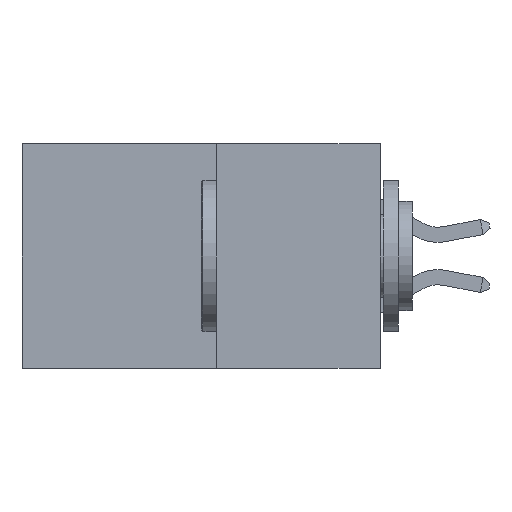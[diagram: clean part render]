
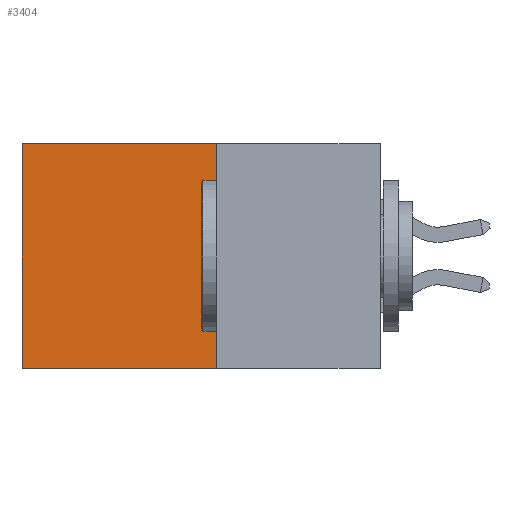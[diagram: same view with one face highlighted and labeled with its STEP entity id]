
A CAD part, left-side view. The second image highlights one B-rep face of the part: STEP entity #3404.
In plain terms, the highlighted planar face has unit normal (-1, 0, 0).
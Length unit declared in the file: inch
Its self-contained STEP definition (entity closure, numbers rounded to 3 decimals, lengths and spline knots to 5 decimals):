
#109 = CARTESIAN_POINT ( 'NONE',  ( 0.277, 0.27, 0. ) ) ;
#290 = DIRECTION ( 'NONE',  ( 0., 1., 0. ) ) ;
#427 = CARTESIAN_POINT ( 'NONE',  ( 0.277, 0.27, -0.37 ) ) ;
#1218 = CARTESIAN_POINT ( 'NONE',  ( 0.277, 0.59, -0.37 ) ) ;
#1622 = CARTESIAN_POINT ( 'NONE',  ( 0.277, 0.59, -0.37 ) ) ;
#3404 = ADVANCED_FACE ( 'NONE', ( #16937 ), #18128, .F. ) ;
#3435 = DIRECTION ( 'NONE',  ( 0., 0., -1. ) ) ;
#5692 = ORIENTED_EDGE ( 'NONE', *, *, #20741, .T. ) ;
#5983 = LINE ( 'NONE', #10711, #20294 ) ;
#6205 = LINE ( 'NONE', #1622, #21079 ) ;
#8335 = ORIENTED_EDGE ( 'NONE', *, *, #9050, .F. ) ;
#8453 = VECTOR ( 'NONE', #15107, 39.37008 ) ;
#9037 = LINE ( 'NONE', #109, #8453 ) ;
#9050 = EDGE_CURVE ( 'NONE', #17726, #15517, #5983, .T. ) ;
#9116 = DIRECTION ( 'NONE',  ( 0., 0., -1. ) ) ;
#9784 = VERTEX_POINT ( 'NONE', #23507 ) ;
#9999 = LINE ( 'NONE', #427, #14352 ) ;
#10662 = EDGE_CURVE ( 'NONE', #15517, #20587, #9999, .T. ) ;
#10711 = CARTESIAN_POINT ( 'NONE',  ( 0.277, 0.27, -0.37 ) ) ;
#13390 = EDGE_CURVE ( 'NONE', #17726, #9784, #9037, .T. ) ;
#13957 = ORIENTED_EDGE ( 'NONE', *, *, #10662, .F. ) ;
#14024 = ORIENTED_EDGE ( 'NONE', *, *, #13390, .T. ) ;
#14352 = VECTOR ( 'NONE', #290, 39.37008 ) ;
#15107 = DIRECTION ( 'NONE',  ( 0., 1., 0. ) ) ;
#15517 = VERTEX_POINT ( 'NONE', #19638 ) ;
#16448 = CARTESIAN_POINT ( 'NONE',  ( 0.277, 0.27, -0.37 ) ) ;
#16605 = DIRECTION ( 'NONE',  ( 0., 0., -1. ) ) ;
#16923 = DIRECTION ( 'NONE',  ( 1., 0., 0. ) ) ;
#16937 = FACE_OUTER_BOUND ( 'NONE', #23700, .T. ) ;
#17726 = VERTEX_POINT ( 'NONE', #18061 ) ;
#18061 = CARTESIAN_POINT ( 'NONE',  ( 0.277, 0.27, 0. ) ) ;
#18128 = PLANE ( 'NONE',  #23372 ) ;
#19638 = CARTESIAN_POINT ( 'NONE',  ( 0.277, 0.27, -0.37 ) ) ;
#20294 = VECTOR ( 'NONE', #3435, 39.37008 ) ;
#20587 = VERTEX_POINT ( 'NONE', #1218 ) ;
#20741 = EDGE_CURVE ( 'NONE', #9784, #20587, #6205, .T. ) ;
#21079 = VECTOR ( 'NONE', #9116, 39.37008 ) ;
#23372 = AXIS2_PLACEMENT_3D ( 'NONE', #16448, #16923, #16605 ) ;
#23507 = CARTESIAN_POINT ( 'NONE',  ( 0.277, 0.59, 0. ) ) ;
#23700 = EDGE_LOOP ( 'NONE', ( #5692, #13957, #8335, #14024 ) ) ;
